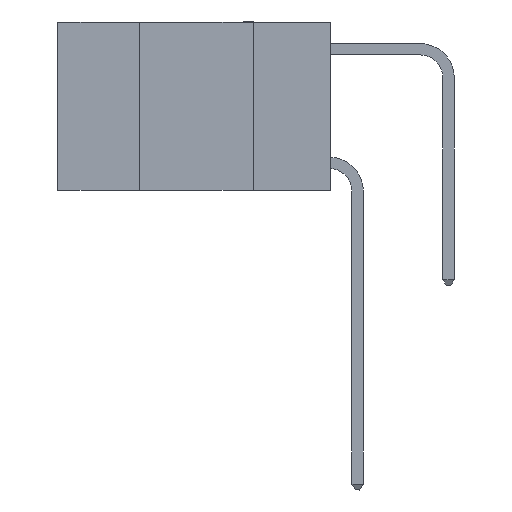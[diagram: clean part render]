
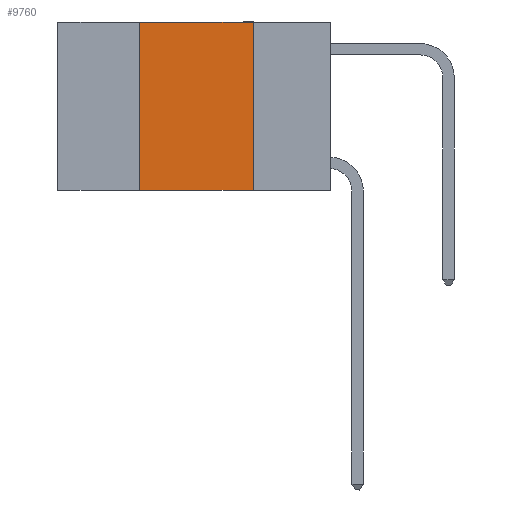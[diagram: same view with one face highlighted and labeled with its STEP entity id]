
A CAD part, left-side view. The second image highlights one B-rep face of the part: STEP entity #9760.
In plain terms, the highlighted planar face has unit normal (-1, 0, 0).
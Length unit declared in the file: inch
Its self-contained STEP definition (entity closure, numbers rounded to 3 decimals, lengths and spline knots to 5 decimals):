
#378 = AXIS2_PLACEMENT_3D ( 'NONE', #11168, #16662, #5638 ) ;
#2992 = DIRECTION ( 'NONE',  ( 0., -1., 0. ) ) ;
#3969 = VERTEX_POINT ( 'NONE', #8147 ) ;
#4470 = ORIENTED_EDGE ( 'NONE', *, *, #8463, .F. ) ;
#4477 = VECTOR ( 'NONE', #14076, 39.37008 ) ;
#4662 = LINE ( 'NONE', #10442, #18773 ) ;
#4673 = CARTESIAN_POINT ( 'NONE',  ( 0., 0.17, -0.37 ) ) ;
#4864 = CARTESIAN_POINT ( 'NONE',  ( 0., 0.17, 0. ) ) ;
#5036 = DIRECTION ( 'NONE',  ( 0., 0., 1. ) ) ;
#5638 = DIRECTION ( 'NONE',  ( 0., 0., -1. ) ) ;
#7428 = VERTEX_POINT ( 'NONE', #18586 ) ;
#8147 = CARTESIAN_POINT ( 'NONE',  ( 0., 0.17, 0. ) ) ;
#8463 = EDGE_CURVE ( 'NONE', #7428, #21035, #14552, .T. ) ;
#9126 = VECTOR ( 'NONE', #5036, 39.37008 ) ;
#9409 = ORIENTED_EDGE ( 'NONE', *, *, #23547, .T. ) ;
#9417 = LINE ( 'NONE', #4864, #4477 ) ;
#9590 = EDGE_LOOP ( 'NONE', ( #16792, #10007, #4470, #9409 ) ) ;
#9760 = ADVANCED_FACE ( 'NONE', ( #16782 ), #16576, .F. ) ;
#10007 = ORIENTED_EDGE ( 'NONE', *, *, #17701, .F. ) ;
#10442 = CARTESIAN_POINT ( 'NONE',  ( 0., 0.6, -0.37 ) ) ;
#11168 = CARTESIAN_POINT ( 'NONE',  ( 0., 0.6, 0. ) ) ;
#12705 = VECTOR ( 'NONE', #15011, 39.37008 ) ;
#13220 = CARTESIAN_POINT ( 'NONE',  ( 0., 0.6, 0. ) ) ;
#13596 = VERTEX_POINT ( 'NONE', #4673 ) ;
#14076 = DIRECTION ( 'NONE',  ( 0., 0., -1. ) ) ;
#14552 = LINE ( 'NONE', #17915, #9126 ) ;
#15011 = DIRECTION ( 'NONE',  ( 0., -1., 0. ) ) ;
#16576 = PLANE ( 'NONE',  #378 ) ;
#16662 = DIRECTION ( 'NONE',  ( 1., 0., 0. ) ) ;
#16782 = FACE_OUTER_BOUND ( 'NONE', #9590, .T. ) ;
#16792 = ORIENTED_EDGE ( 'NONE', *, *, #19822, .F. ) ;
#17701 = EDGE_CURVE ( 'NONE', #21035, #3969, #21749, .T. ) ;
#17915 = CARTESIAN_POINT ( 'NONE',  ( 0., 0.42, 0. ) ) ;
#18586 = CARTESIAN_POINT ( 'NONE',  ( 0., 0.42, -0.37 ) ) ;
#18773 = VECTOR ( 'NONE', #2992, 39.37008 ) ;
#19440 = CARTESIAN_POINT ( 'NONE',  ( 0., 0.42, 0. ) ) ;
#19822 = EDGE_CURVE ( 'NONE', #3969, #13596, #9417, .T. ) ;
#21035 = VERTEX_POINT ( 'NONE', #19440 ) ;
#21749 = LINE ( 'NONE', #13220, #12705 ) ;
#23547 = EDGE_CURVE ( 'NONE', #7428, #13596, #4662, .T. ) ;
